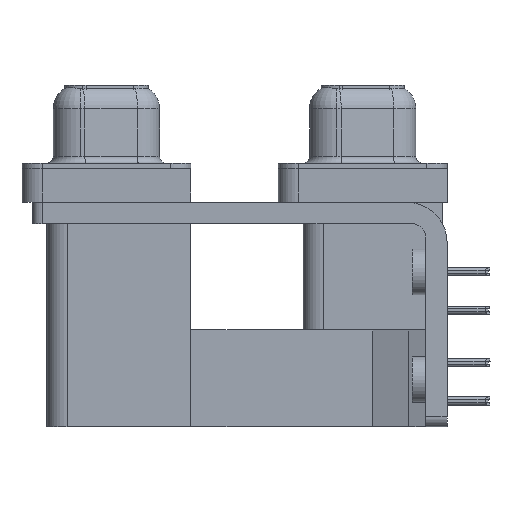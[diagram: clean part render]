
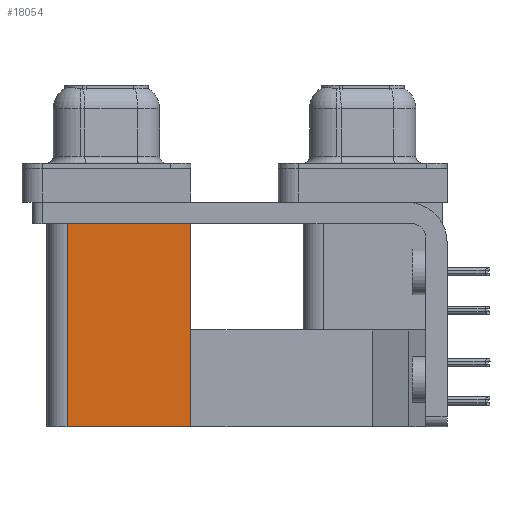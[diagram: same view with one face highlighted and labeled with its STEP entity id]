
A CAD part, left-side view. The second image highlights one B-rep face of the part: STEP entity #18054.
In plain terms, the highlighted planar face has unit normal (-1, 0, 0).
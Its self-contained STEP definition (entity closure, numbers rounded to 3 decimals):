
#389 = EDGE_LOOP ( 'NONE', ( #23350, #42018, #4456, #44092 ) ) ;
#652 = LINE ( 'NONE', #4466, #42263 ) ;
#1338 = VERTEX_POINT ( 'NONE', #2808 ) ;
#1814 = EDGE_CURVE ( 'NONE', #3942, #1338, #2538, .T. ) ;
#2266 = CARTESIAN_POINT ( 'NONE',  ( 3.79, 12.775, -19.2 ) ) ;
#2538 = LINE ( 'NONE', #19662, #31260 ) ;
#2808 = CARTESIAN_POINT ( 'NONE',  ( 3.79, 21.975, -2.5 ) ) ;
#3942 = VERTEX_POINT ( 'NONE', #11602 ) ;
#4309 = EDGE_CURVE ( 'NONE', #32641, #8644, #16702, .T. ) ;
#4456 = ORIENTED_EDGE ( 'NONE', *, *, #24877, .F. ) ;
#4466 = CARTESIAN_POINT ( 'NONE',  ( 3.79, 12.775, -19.2 ) ) ;
#6519 = CARTESIAN_POINT ( 'NONE',  ( 3.79, 12.775, -19.2 ) ) ;
#6639 = CARTESIAN_POINT ( 'NONE',  ( 3.79, 12.775, -2.5 ) ) ;
#8644 = VERTEX_POINT ( 'NONE', #6639 ) ;
#8867 = DIRECTION ( 'NONE',  ( 0., 0., 1. ) ) ;
#10117 = DIRECTION ( 'NONE',  ( 1., 0., 0. ) ) ;
#11602 = CARTESIAN_POINT ( 'NONE',  ( 3.79, 21.975, -19.2 ) ) ;
#11995 = CARTESIAN_POINT ( 'NONE',  ( 3.79, 12.775, -19.2 ) ) ;
#16035 = DIRECTION ( 'NONE',  ( 0., 0., 1. ) ) ;
#16702 = LINE ( 'NONE', #2266, #33724 ) ;
#16758 = CARTESIAN_POINT ( 'NONE',  ( 3.79, 12.775, -2.5 ) ) ;
#17785 = DIRECTION ( 'NONE',  ( 0., 1., 0. ) ) ;
#18054 = ADVANCED_FACE ( 'NONE', ( #34449 ), #37594, .F. ) ;
#18223 = DIRECTION ( 'NONE',  ( 0., 1., 0. ) ) ;
#19662 = CARTESIAN_POINT ( 'NONE',  ( 3.79, 21.975, -19.2 ) ) ;
#23350 = ORIENTED_EDGE ( 'NONE', *, *, #32421, .T. ) ;
#23730 = DIRECTION ( 'NONE',  ( 0., 1., 0. ) ) ;
#24877 = EDGE_CURVE ( 'NONE', #32641, #3942, #652, .T. ) ;
#31260 = VECTOR ( 'NONE', #8867, 1000. ) ;
#32421 = EDGE_CURVE ( 'NONE', #8644, #1338, #33865, .T. ) ;
#32641 = VERTEX_POINT ( 'NONE', #11995 ) ;
#33724 = VECTOR ( 'NONE', #16035, 1000. ) ;
#33782 = AXIS2_PLACEMENT_3D ( 'NONE', #6519, #10117, #17785 ) ;
#33865 = LINE ( 'NONE', #16758, #44233 ) ;
#34449 = FACE_OUTER_BOUND ( 'NONE', #389, .T. ) ;
#37594 = PLANE ( 'NONE',  #33782 ) ;
#42018 = ORIENTED_EDGE ( 'NONE', *, *, #1814, .F. ) ;
#42263 = VECTOR ( 'NONE', #18223, 1000. ) ;
#44092 = ORIENTED_EDGE ( 'NONE', *, *, #4309, .T. ) ;
#44233 = VECTOR ( 'NONE', #23730, 1000. ) ;
